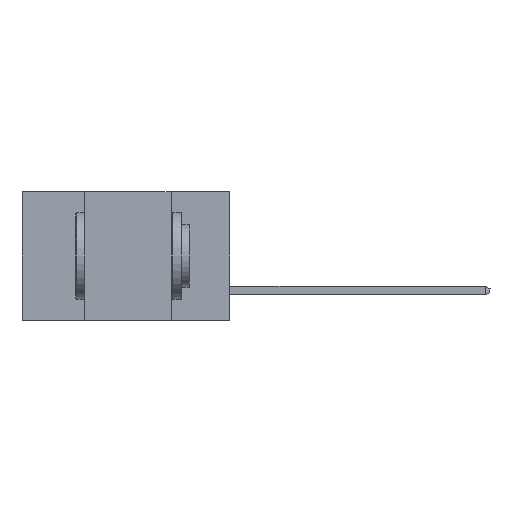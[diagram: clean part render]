
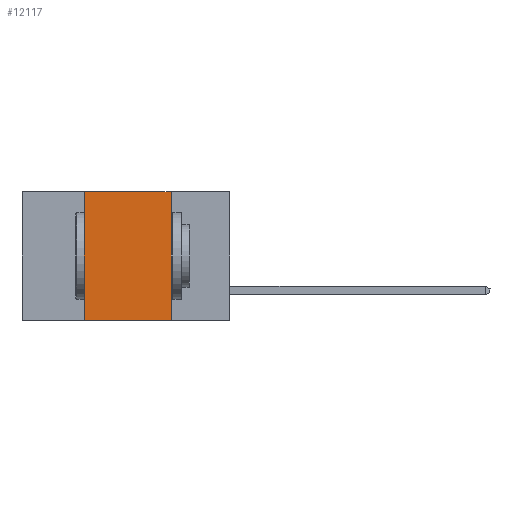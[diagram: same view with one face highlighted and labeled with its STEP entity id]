
A CAD part, left-side view. The second image highlights one B-rep face of the part: STEP entity #12117.
In plain terms, the highlighted planar face has unit normal (-1, 0, 0).
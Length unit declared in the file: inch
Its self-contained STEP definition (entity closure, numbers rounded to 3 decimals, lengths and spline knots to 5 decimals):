
#414 = LINE ( 'NONE', #13235, #3648 ) ;
#612 = EDGE_CURVE ( 'NONE', #10485, #4902, #12909, .T. ) ;
#1436 = DIRECTION ( 'NONE',  ( 0., -1., 0. ) ) ;
#1717 = ORIENTED_EDGE ( 'NONE', *, *, #14626, .F. ) ;
#1893 = AXIS2_PLACEMENT_3D ( 'NONE', #15660, #11692, #11459 ) ;
#2349 = CARTESIAN_POINT ( 'NONE',  ( 0., 0.6, 0. ) ) ;
#2594 = VECTOR ( 'NONE', #1436, 39.37008 ) ;
#3002 = DIRECTION ( 'NONE',  ( 0., -1., 0. ) ) ;
#3648 = VECTOR ( 'NONE', #9208, 39.37008 ) ;
#3826 = ORIENTED_EDGE ( 'NONE', *, *, #612, .T. ) ;
#3886 = FACE_OUTER_BOUND ( 'NONE', #4206, .T. ) ;
#4206 = EDGE_LOOP ( 'NONE', ( #14158, #16674, #1717, #3826 ) ) ;
#4335 = CARTESIAN_POINT ( 'NONE',  ( 0., 0.17, 0. ) ) ;
#4395 = EDGE_CURVE ( 'NONE', #11784, #4902, #10168, .T. ) ;
#4902 = VERTEX_POINT ( 'NONE', #7497 ) ;
#6027 = PLANE ( 'NONE',  #1893 ) ;
#6298 = VERTEX_POINT ( 'NONE', #12950 ) ;
#7497 = CARTESIAN_POINT ( 'NONE',  ( 0., 0.17, -0.37 ) ) ;
#7557 = LINE ( 'NONE', #2349, #2594 ) ;
#9208 = DIRECTION ( 'NONE',  ( 0., 0., 1. ) ) ;
#10168 = LINE ( 'NONE', #4335, #11458 ) ;
#10485 = VERTEX_POINT ( 'NONE', #11201 ) ;
#11201 = CARTESIAN_POINT ( 'NONE',  ( 0., 0.42, -0.37 ) ) ;
#11207 = DIRECTION ( 'NONE',  ( 0., 0., -1. ) ) ;
#11458 = VECTOR ( 'NONE', #11207, 39.37008 ) ;
#11459 = DIRECTION ( 'NONE',  ( 0., 0., -1. ) ) ;
#11692 = DIRECTION ( 'NONE',  ( 1., 0., 0. ) ) ;
#11784 = VERTEX_POINT ( 'NONE', #13614 ) ;
#11965 = EDGE_CURVE ( 'NONE', #6298, #11784, #7557, .T. ) ;
#12117 = ADVANCED_FACE ( 'NONE', ( #3886 ), #6027, .F. ) ;
#12176 = CARTESIAN_POINT ( 'NONE',  ( 0., 0.6, -0.37 ) ) ;
#12909 = LINE ( 'NONE', #12176, #15030 ) ;
#12950 = CARTESIAN_POINT ( 'NONE',  ( 0., 0.42, 0. ) ) ;
#13235 = CARTESIAN_POINT ( 'NONE',  ( 0., 0.42, 0. ) ) ;
#13614 = CARTESIAN_POINT ( 'NONE',  ( 0., 0.17, 0. ) ) ;
#14158 = ORIENTED_EDGE ( 'NONE', *, *, #4395, .F. ) ;
#14626 = EDGE_CURVE ( 'NONE', #10485, #6298, #414, .T. ) ;
#15030 = VECTOR ( 'NONE', #3002, 39.37008 ) ;
#15660 = CARTESIAN_POINT ( 'NONE',  ( 0., 0.6, 0. ) ) ;
#16674 = ORIENTED_EDGE ( 'NONE', *, *, #11965, .F. ) ;
